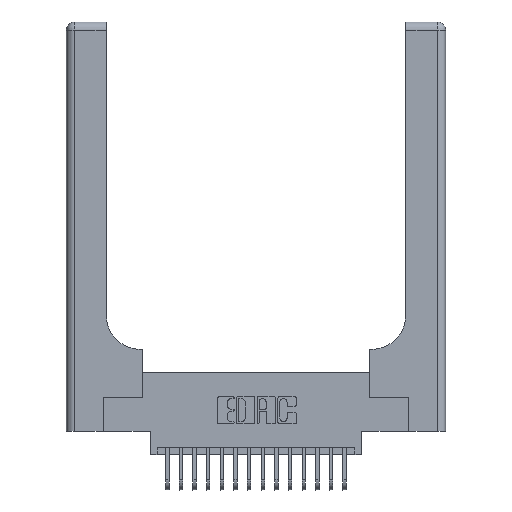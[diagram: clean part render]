
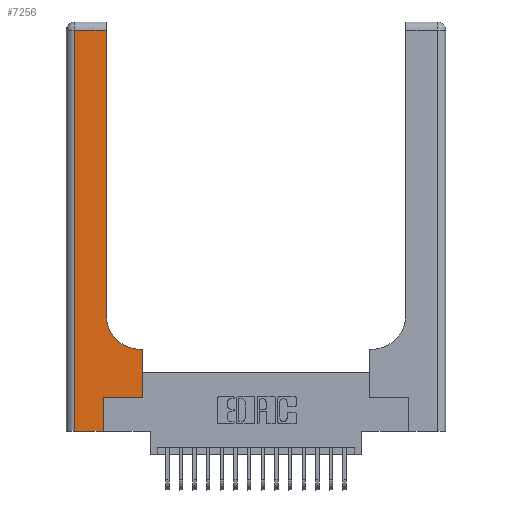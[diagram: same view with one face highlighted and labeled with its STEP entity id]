
A CAD part, top view. The second image highlights one B-rep face of the part: STEP entity #7256.
In plain terms, the highlighted planar face has unit normal (0, 0, 1).
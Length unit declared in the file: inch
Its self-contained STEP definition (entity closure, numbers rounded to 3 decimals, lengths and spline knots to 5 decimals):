
#566 = EDGE_CURVE ( 'NONE', #19548, #3911, #9290, .T. ) ;
#610 = EDGE_CURVE ( 'NONE', #2254, #18552, #12369, .T. ) ;
#924 = VECTOR ( 'NONE', #15460, 39.37008 ) ;
#1236 = FACE_OUTER_BOUND ( 'NONE', #5793, .T. ) ;
#1464 = EDGE_CURVE ( 'NONE', #18552, #19548, #7134, .T. ) ;
#2038 = ORIENTED_EDGE ( 'NONE', *, *, #5722, .T. ) ;
#2254 = VERTEX_POINT ( 'NONE', #12935 ) ;
#2835 = CARTESIAN_POINT ( 'NONE',  ( 0.2915, 0.6, 0.37 ) ) ;
#3016 = AXIS2_PLACEMENT_3D ( 'NONE', #15858, #17361, #8296 ) ;
#3139 = EDGE_CURVE ( 'NONE', #5293, #11494, #9078, .T. ) ;
#3911 = VERTEX_POINT ( 'NONE', #6741 ) ;
#4659 = LINE ( 'NONE', #6983, #16307 ) ;
#5081 = ORIENTED_EDGE ( 'NONE', *, *, #15787, .T. ) ;
#5241 = VECTOR ( 'NONE', #12485, 39.37008 ) ;
#5293 = VERTEX_POINT ( 'NONE', #18615 ) ;
#5294 = DIRECTION ( 'NONE',  ( 0., -1., 0. ) ) ;
#5523 = ORIENTED_EDGE ( 'NONE', *, *, #12473, .T. ) ;
#5722 = EDGE_CURVE ( 'NONE', #15146, #5977, #11329, .T. ) ;
#5793 = EDGE_LOOP ( 'NONE', ( #6707, #8906, #11251, #2038, #13356, #9528, #5523, #5081, #9606 ) ) ;
#5829 = CARTESIAN_POINT ( 'NONE',  ( 0.269, 0., 0.37 ) ) ;
#5977 = VERTEX_POINT ( 'NONE', #5829 ) ;
#6634 = VECTOR ( 'NONE', #10632, 39.37008 ) ;
#6707 = ORIENTED_EDGE ( 'NONE', *, *, #1464, .T. ) ;
#6741 = CARTESIAN_POINT ( 'NONE',  ( 0.06, 2.94, 0.37 ) ) ;
#6983 = CARTESIAN_POINT ( 'NONE',  ( 0.269, 0., 0.37 ) ) ;
#7134 = LINE ( 'NONE', #12161, #6634 ) ;
#7256 = ADVANCED_FACE ( 'NONE', ( #1236 ), #8237, .F. ) ;
#7294 = EDGE_CURVE ( 'NONE', #3911, #15146, #16499, .T. ) ;
#7817 = LINE ( 'NONE', #2835, #15409 ) ;
#8237 = PLANE ( 'NONE',  #3016 ) ;
#8296 = DIRECTION ( 'NONE',  ( -1., 0., 0. ) ) ;
#8400 = CARTESIAN_POINT ( 'NONE',  ( 0.5585, 0.6, 0.37 ) ) ;
#8435 = VECTOR ( 'NONE', #5294, 39.37008 ) ;
#8906 = ORIENTED_EDGE ( 'NONE', *, *, #566, .T. ) ;
#9078 = LINE ( 'NONE', #12401, #924 ) ;
#9290 = LINE ( 'NONE', #12547, #5241 ) ;
#9388 = CARTESIAN_POINT ( 'NONE',  ( 0.2915, 0.85, 0.37 ) ) ;
#9528 = ORIENTED_EDGE ( 'NONE', *, *, #3139, .T. ) ;
#9606 = ORIENTED_EDGE ( 'NONE', *, *, #610, .T. ) ;
#10537 = CARTESIAN_POINT ( 'NONE',  ( 0.06, 0., 0.37 ) ) ;
#10632 = DIRECTION ( 'NONE',  ( 0., 1., 0. ) ) ;
#10709 = EDGE_CURVE ( 'NONE', #5977, #5293, #4659, .T. ) ;
#11251 = ORIENTED_EDGE ( 'NONE', *, *, #7294, .T. ) ;
#11329 = LINE ( 'NONE', #17168, #11831 ) ;
#11494 = VERTEX_POINT ( 'NONE', #11807 ) ;
#11807 = CARTESIAN_POINT ( 'NONE',  ( 0.5585, 0.25, 0.37 ) ) ;
#11831 = VECTOR ( 'NONE', #14208, 39.37008 ) ;
#12056 = DIRECTION ( 'NONE',  ( -1., 0., 0. ) ) ;
#12161 = CARTESIAN_POINT ( 'NONE',  ( 0.2915, 3., 0.37 ) ) ;
#12187 = VECTOR ( 'NONE', #14109, 39.37008 ) ;
#12369 = CIRCLE ( 'NONE', #14541, 0.25 ) ;
#12401 = CARTESIAN_POINT ( 'NONE',  ( 0.269, 0.25, 0.37 ) ) ;
#12473 = EDGE_CURVE ( 'NONE', #11494, #14356, #16227, .T. ) ;
#12485 = DIRECTION ( 'NONE',  ( -1., 0., 0. ) ) ;
#12547 = CARTESIAN_POINT ( 'NONE',  ( 0., 2.94, 0.37 ) ) ;
#12574 = CARTESIAN_POINT ( 'NONE',  ( 0.5585, 0.25, 0.37 ) ) ;
#12871 = CARTESIAN_POINT ( 'NONE',  ( 0.06, 3., 0.37 ) ) ;
#12935 = CARTESIAN_POINT ( 'NONE',  ( 0.5415, 0.6, 0.37 ) ) ;
#13356 = ORIENTED_EDGE ( 'NONE', *, *, #10709, .T. ) ;
#13634 = DIRECTION ( 'NONE',  ( 1., 0., 0. ) ) ;
#13658 = DIRECTION ( 'NONE',  ( 0., 0., -1. ) ) ;
#13707 = CARTESIAN_POINT ( 'NONE',  ( 0.5415, 0.85, 0.37 ) ) ;
#14109 = DIRECTION ( 'NONE',  ( 0., 1., 0. ) ) ;
#14208 = DIRECTION ( 'NONE',  ( 1., 0., 0. ) ) ;
#14356 = VERTEX_POINT ( 'NONE', #8400 ) ;
#14541 = AXIS2_PLACEMENT_3D ( 'NONE', #13707, #13658, #13634 ) ;
#14542 = DIRECTION ( 'NONE',  ( 0., 1., 0. ) ) ;
#15146 = VERTEX_POINT ( 'NONE', #10537 ) ;
#15409 = VECTOR ( 'NONE', #12056, 39.37008 ) ;
#15460 = DIRECTION ( 'NONE',  ( 1., 0., 0. ) ) ;
#15642 = CARTESIAN_POINT ( 'NONE',  ( 0.2915, 2.94, 0.37 ) ) ;
#15787 = EDGE_CURVE ( 'NONE', #14356, #2254, #7817, .T. ) ;
#15858 = CARTESIAN_POINT ( 'NONE',  ( 0., 3., 0.37 ) ) ;
#16227 = LINE ( 'NONE', #12574, #12187 ) ;
#16307 = VECTOR ( 'NONE', #14542, 39.37008 ) ;
#16499 = LINE ( 'NONE', #12871, #8435 ) ;
#17168 = CARTESIAN_POINT ( 'NONE',  ( 0., 0., 0.37 ) ) ;
#17361 = DIRECTION ( 'NONE',  ( 0., 0., -1. ) ) ;
#18552 = VERTEX_POINT ( 'NONE', #9388 ) ;
#18615 = CARTESIAN_POINT ( 'NONE',  ( 0.269, 0.25, 0.37 ) ) ;
#19548 = VERTEX_POINT ( 'NONE', #15642 ) ;
